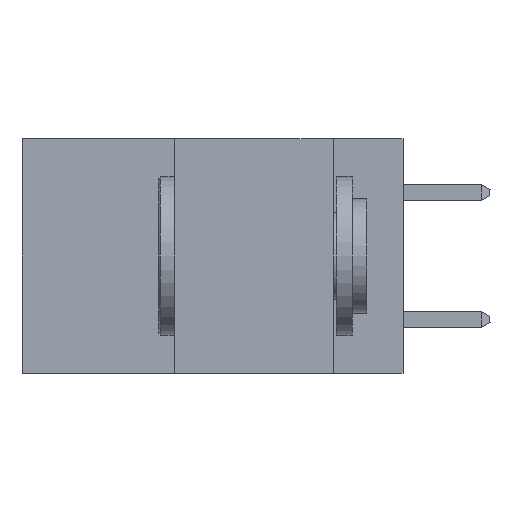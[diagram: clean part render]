
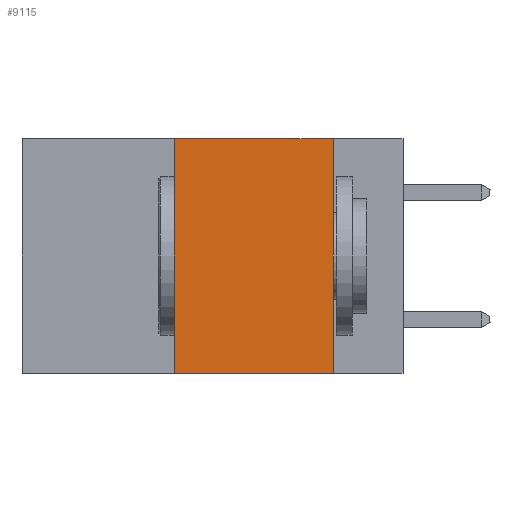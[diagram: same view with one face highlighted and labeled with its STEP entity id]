
A CAD part, left-side view. The second image highlights one B-rep face of the part: STEP entity #9115.
In plain terms, the highlighted planar face has unit normal (-1, 0, 0).
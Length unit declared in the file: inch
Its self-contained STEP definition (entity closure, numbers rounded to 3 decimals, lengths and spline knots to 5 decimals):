
#66 = LINE ( 'NONE', #28159, #27313 ) ;
#593 = ORIENTED_EDGE ( 'NONE', *, *, #44903, .T. ) ;
#598 = EDGE_CURVE ( 'NONE', #14764, #7789, #23246, .T. ) ;
#3621 = VERTEX_POINT ( 'NONE', #23937 ) ;
#4018 = CARTESIAN_POINT ( 'NONE',  ( 0., 0.11, 0. ) ) ;
#5410 = VECTOR ( 'NONE', #38596, 39.37008 ) ;
#7789 = VERTEX_POINT ( 'NONE', #26197 ) ;
#9115 = ADVANCED_FACE ( 'NONE', ( #29719 ), #43739, .F. ) ;
#10298 = CARTESIAN_POINT ( 'NONE',  ( 0., 0.6, -0.37 ) ) ;
#11369 = DIRECTION ( 'NONE',  ( 1., 0., 0. ) ) ;
#13786 = VECTOR ( 'NONE', #29525, 39.37008 ) ;
#14764 = VERTEX_POINT ( 'NONE', #26308 ) ;
#18187 = VERTEX_POINT ( 'NONE', #4018 ) ;
#19542 = ORIENTED_EDGE ( 'NONE', *, *, #31045, .F. ) ;
#23246 = LINE ( 'NONE', #29676, #13786 ) ;
#23937 = CARTESIAN_POINT ( 'NONE',  ( 0., 0.11, -0.37 ) ) ;
#25477 = DIRECTION ( 'NONE',  ( 0., 0., -1. ) ) ;
#26197 = CARTESIAN_POINT ( 'NONE',  ( 0., 0.36, 0. ) ) ;
#26308 = CARTESIAN_POINT ( 'NONE',  ( 0., 0.36, -0.37 ) ) ;
#27313 = VECTOR ( 'NONE', #35355, 39.37008 ) ;
#27580 = ORIENTED_EDGE ( 'NONE', *, *, #598, .F. ) ;
#28159 = CARTESIAN_POINT ( 'NONE',  ( 0., 0.11, 0. ) ) ;
#28777 = EDGE_CURVE ( 'NONE', #18187, #3621, #66, .T. ) ;
#29525 = DIRECTION ( 'NONE',  ( 0., 0., 1. ) ) ;
#29676 = CARTESIAN_POINT ( 'NONE',  ( 0., 0.36, 0. ) ) ;
#29719 = FACE_OUTER_BOUND ( 'NONE', #42509, .T. ) ;
#31045 = EDGE_CURVE ( 'NONE', #7789, #18187, #34323, .T. ) ;
#31122 = VECTOR ( 'NONE', #45634, 39.37008 ) ;
#31400 = CARTESIAN_POINT ( 'NONE',  ( 0., 0.6, 0. ) ) ;
#34323 = LINE ( 'NONE', #31400, #5410 ) ;
#35355 = DIRECTION ( 'NONE',  ( 0., 0., -1. ) ) ;
#35618 = AXIS2_PLACEMENT_3D ( 'NONE', #43266, #11369, #25477 ) ;
#37876 = LINE ( 'NONE', #10298, #31122 ) ;
#38596 = DIRECTION ( 'NONE',  ( 0., -1., 0. ) ) ;
#38690 = ORIENTED_EDGE ( 'NONE', *, *, #28777, .F. ) ;
#42509 = EDGE_LOOP ( 'NONE', ( #38690, #19542, #27580, #593 ) ) ;
#43266 = CARTESIAN_POINT ( 'NONE',  ( 0., 0.6, 0. ) ) ;
#43739 = PLANE ( 'NONE',  #35618 ) ;
#44903 = EDGE_CURVE ( 'NONE', #14764, #3621, #37876, .T. ) ;
#45634 = DIRECTION ( 'NONE',  ( 0., -1., 0. ) ) ;
